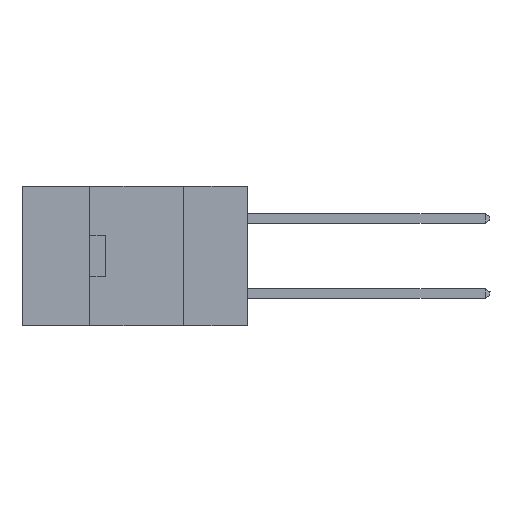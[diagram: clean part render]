
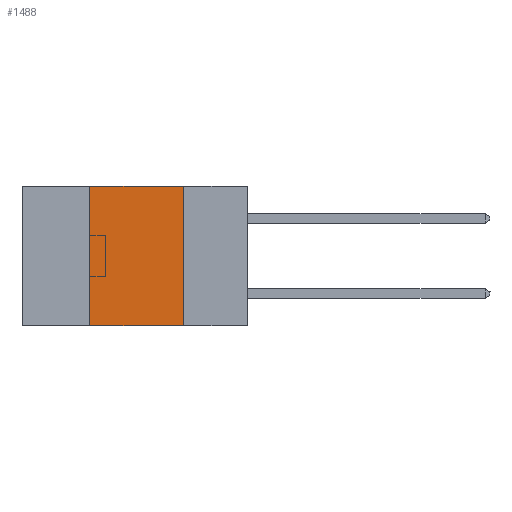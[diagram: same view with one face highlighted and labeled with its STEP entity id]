
A CAD part, left-side view. The second image highlights one B-rep face of the part: STEP entity #1488.
In plain terms, the highlighted planar face has unit normal (-1, 0, 0).
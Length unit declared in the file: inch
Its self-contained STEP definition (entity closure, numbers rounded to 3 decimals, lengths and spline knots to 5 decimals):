
#1392 = VERTEX_POINT ( 'NONE', #4473 ) ;
#1488 = ADVANCED_FACE ( 'NONE', ( #14316 ), #2827, .F. ) ;
#2635 = DIRECTION ( 'NONE',  ( 0., 0., -1. ) ) ;
#2660 = DIRECTION ( 'NONE',  ( 1., 0., 0. ) ) ;
#2795 = CARTESIAN_POINT ( 'NONE',  ( 0., 0.6, 0. ) ) ;
#2827 = PLANE ( 'NONE',  #26425 ) ;
#4160 = CARTESIAN_POINT ( 'NONE',  ( 0., 0.17, -0.37 ) ) ;
#4460 = CARTESIAN_POINT ( 'NONE',  ( 0., 0.6, 0. ) ) ;
#4473 = CARTESIAN_POINT ( 'NONE',  ( 0., 0.17, 0. ) ) ;
#4527 = VERTEX_POINT ( 'NONE', #15156 ) ;
#5415 = CARTESIAN_POINT ( 'NONE',  ( 0., 0.17, -0.37 ) ) ;
#6400 = VECTOR ( 'NONE', #20301, 39.37008 ) ;
#8320 = EDGE_LOOP ( 'NONE', ( #24634, #24660, #23658, #9342 ) ) ;
#8896 = LINE ( 'NONE', #17277, #20148 ) ;
#9342 = ORIENTED_EDGE ( 'NONE', *, *, #26511, .T. ) ;
#10452 = LINE ( 'NONE', #4160, #15733 ) ;
#11932 = EDGE_CURVE ( 'NONE', #1392, #20267, #10452, .T. ) ;
#13812 = LINE ( 'NONE', #20400, #6400 ) ;
#14316 = FACE_OUTER_BOUND ( 'NONE', #8320, .T. ) ;
#15034 = DIRECTION ( 'NONE',  ( 0., -1., 0. ) ) ;
#15156 = CARTESIAN_POINT ( 'NONE',  ( 0., 0.42, 0. ) ) ;
#15733 = VECTOR ( 'NONE', #24320, 39.37008 ) ;
#17277 = CARTESIAN_POINT ( 'NONE',  ( 0., 0.6, -0.37 ) ) ;
#17952 = DIRECTION ( 'NONE',  ( 0., -1., 0. ) ) ;
#20148 = VECTOR ( 'NONE', #15034, 39.37008 ) ;
#20267 = VERTEX_POINT ( 'NONE', #5415 ) ;
#20301 = DIRECTION ( 'NONE',  ( 0., 0., 1. ) ) ;
#20400 = CARTESIAN_POINT ( 'NONE',  ( 0., 0.42, -0.37 ) ) ;
#20481 = LINE ( 'NONE', #4460, #26325 ) ;
#22529 = CARTESIAN_POINT ( 'NONE',  ( 0., 0.42, -0.37 ) ) ;
#23658 = ORIENTED_EDGE ( 'NONE', *, *, #26797, .F. ) ;
#24320 = DIRECTION ( 'NONE',  ( 0., 0., -1. ) ) ;
#24634 = ORIENTED_EDGE ( 'NONE', *, *, #11932, .F. ) ;
#24660 = ORIENTED_EDGE ( 'NONE', *, *, #26708, .F. ) ;
#26325 = VECTOR ( 'NONE', #17952, 39.37008 ) ;
#26425 = AXIS2_PLACEMENT_3D ( 'NONE', #2795, #2660, #2635 ) ;
#26511 = EDGE_CURVE ( 'NONE', #28206, #20267, #8896, .T. ) ;
#26708 = EDGE_CURVE ( 'NONE', #4527, #1392, #20481, .T. ) ;
#26797 = EDGE_CURVE ( 'NONE', #28206, #4527, #13812, .T. ) ;
#28206 = VERTEX_POINT ( 'NONE', #22529 ) ;
